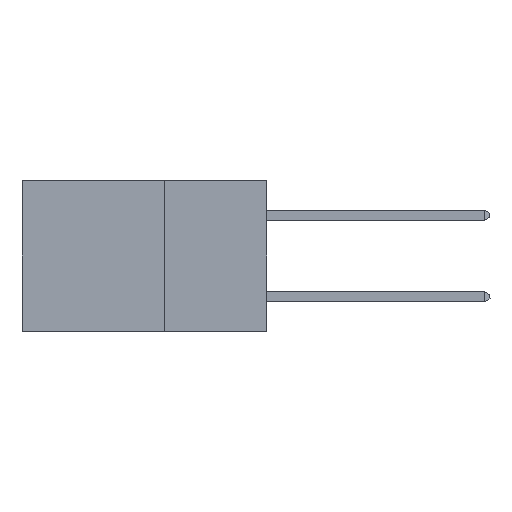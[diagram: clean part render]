
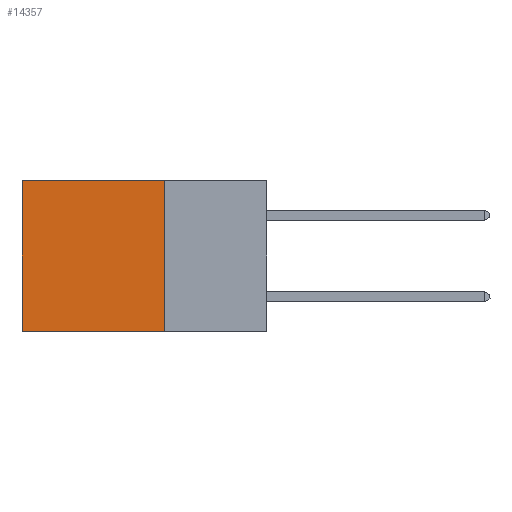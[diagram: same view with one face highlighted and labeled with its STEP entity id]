
A CAD part, left-side view. The second image highlights one B-rep face of the part: STEP entity #14357.
In plain terms, the highlighted planar face has unit normal (-1, 0, 0).
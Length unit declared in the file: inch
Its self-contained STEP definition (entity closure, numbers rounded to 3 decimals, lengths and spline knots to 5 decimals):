
#120 = EDGE_CURVE ( 'NONE', #12661, #9525, #12013, .T. ) ;
#356 = CARTESIAN_POINT ( 'NONE',  ( 0.2875, 0.6, 0. ) ) ;
#1043 = VECTOR ( 'NONE', #15453, 39.37008 ) ;
#2044 = CARTESIAN_POINT ( 'NONE',  ( 0.2875, 0.25, 0. ) ) ;
#2140 = AXIS2_PLACEMENT_3D ( 'NONE', #9769, #13539, #7180 ) ;
#3592 = LINE ( 'NONE', #14098, #10484 ) ;
#4308 = EDGE_CURVE ( 'NONE', #12661, #7864, #8051, .T. ) ;
#4565 = PLANE ( 'NONE',  #2140 ) ;
#4851 = LINE ( 'NONE', #10550, #1043 ) ;
#5030 = VECTOR ( 'NONE', #14838, 39.37008 ) ;
#5676 = ORIENTED_EDGE ( 'NONE', *, *, #15942, .T. ) ;
#7180 = DIRECTION ( 'NONE',  ( 0., 0., -1. ) ) ;
#7864 = VERTEX_POINT ( 'NONE', #356 ) ;
#8051 = LINE ( 'NONE', #13581, #5030 ) ;
#8426 = EDGE_LOOP ( 'NONE', ( #5676, #13736, #11462, #14513 ) ) ;
#9525 = VERTEX_POINT ( 'NONE', #10164 ) ;
#9769 = CARTESIAN_POINT ( 'NONE',  ( 0.2875, 0.25, 0. ) ) ;
#10164 = CARTESIAN_POINT ( 'NONE',  ( 0.2875, 0.25, -0.37 ) ) ;
#10484 = VECTOR ( 'NONE', #15556, 39.37008 ) ;
#10550 = CARTESIAN_POINT ( 'NONE',  ( 0.2875, 0.6, 0. ) ) ;
#11462 = ORIENTED_EDGE ( 'NONE', *, *, #120, .F. ) ;
#12013 = LINE ( 'NONE', #2044, #16630 ) ;
#12661 = VERTEX_POINT ( 'NONE', #13766 ) ;
#13539 = DIRECTION ( 'NONE',  ( 1., 0., 0. ) ) ;
#13581 = CARTESIAN_POINT ( 'NONE',  ( 0.2875, 0.25, 0. ) ) ;
#13736 = ORIENTED_EDGE ( 'NONE', *, *, #16521, .F. ) ;
#13766 = CARTESIAN_POINT ( 'NONE',  ( 0.2875, 0.25, 0. ) ) ;
#14098 = CARTESIAN_POINT ( 'NONE',  ( 0.2875, 0.25, -0.37 ) ) ;
#14357 = ADVANCED_FACE ( 'NONE', ( #16579 ), #4565, .F. ) ;
#14513 = ORIENTED_EDGE ( 'NONE', *, *, #4308, .T. ) ;
#14838 = DIRECTION ( 'NONE',  ( 0., 1., 0. ) ) ;
#15453 = DIRECTION ( 'NONE',  ( 0., 0., -1. ) ) ;
#15556 = DIRECTION ( 'NONE',  ( 0., 1., 0. ) ) ;
#15942 = EDGE_CURVE ( 'NONE', #7864, #16171, #4851, .T. ) ;
#16013 = CARTESIAN_POINT ( 'NONE',  ( 0.2875, 0.6, -0.37 ) ) ;
#16171 = VERTEX_POINT ( 'NONE', #16013 ) ;
#16248 = DIRECTION ( 'NONE',  ( 0., 0., -1. ) ) ;
#16521 = EDGE_CURVE ( 'NONE', #9525, #16171, #3592, .T. ) ;
#16579 = FACE_OUTER_BOUND ( 'NONE', #8426, .T. ) ;
#16630 = VECTOR ( 'NONE', #16248, 39.37008 ) ;
